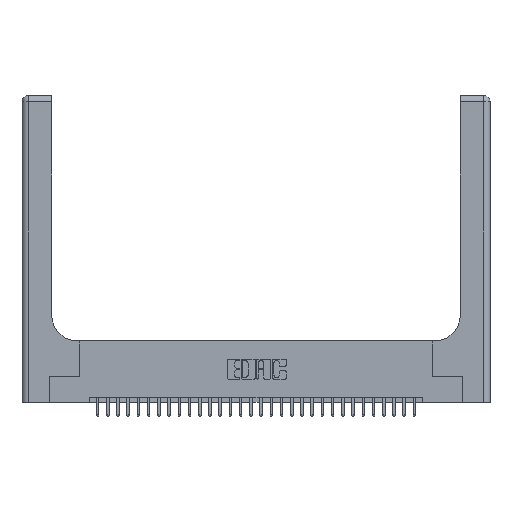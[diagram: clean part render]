
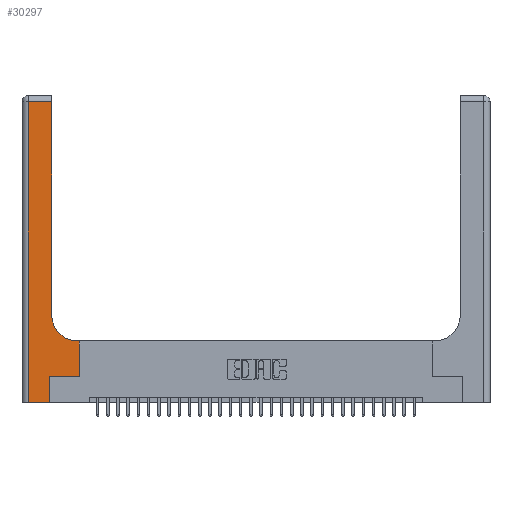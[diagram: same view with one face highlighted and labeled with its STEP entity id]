
A CAD part, top view. The second image highlights one B-rep face of the part: STEP entity #30297.
In plain terms, the highlighted planar face has unit normal (0, 0, 1).
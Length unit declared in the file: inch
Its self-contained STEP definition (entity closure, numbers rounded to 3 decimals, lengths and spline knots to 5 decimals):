
#451 = CARTESIAN_POINT ( 'NONE',  ( 0.06, 0., 0.37 ) ) ;
#680 = EDGE_CURVE ( 'NONE', #16066, #14403, #4061, .T. ) ;
#1610 = CARTESIAN_POINT ( 'NONE',  ( 0., 3., 0.37 ) ) ;
#1974 = ORIENTED_EDGE ( 'NONE', *, *, #22517, .T. ) ;
#2512 = CARTESIAN_POINT ( 'NONE',  ( 0.269, 0.25, 0.37 ) ) ;
#2565 = EDGE_CURVE ( 'NONE', #5691, #30309, #18176, .T. ) ;
#2757 = VERTEX_POINT ( 'NONE', #10152 ) ;
#2891 = EDGE_CURVE ( 'NONE', #23864, #22957, #27853, .T. ) ;
#3194 = VECTOR ( 'NONE', #7421, 39.37008 ) ;
#3577 = EDGE_CURVE ( 'NONE', #22957, #16066, #4499, .T. ) ;
#3822 = FACE_OUTER_BOUND ( 'NONE', #22578, .T. ) ;
#4061 = LINE ( 'NONE', #12243, #22825 ) ;
#4499 = CIRCLE ( 'NONE', #15619, 0.25 ) ;
#4752 = LINE ( 'NONE', #30649, #11666 ) ;
#5093 = DIRECTION ( 'NONE',  ( 0., 1., 0. ) ) ;
#5436 = ORIENTED_EDGE ( 'NONE', *, *, #22120, .T. ) ;
#5691 = VERTEX_POINT ( 'NONE', #451 ) ;
#6523 = EDGE_CURVE ( 'NONE', #2757, #23864, #14977, .T. ) ;
#6579 = DIRECTION ( 'NONE',  ( -1., 0., 0. ) ) ;
#7201 = DIRECTION ( 'NONE',  ( 1., 0., 0. ) ) ;
#7208 = CARTESIAN_POINT ( 'NONE',  ( 0.2915, 0.6, 0.37 ) ) ;
#7421 = DIRECTION ( 'NONE',  ( 1., 0., 0. ) ) ;
#7479 = ORIENTED_EDGE ( 'NONE', *, *, #6523, .T. ) ;
#7613 = VECTOR ( 'NONE', #19084, 39.37008 ) ;
#8499 = VECTOR ( 'NONE', #5093, 39.37008 ) ;
#9966 = DIRECTION ( 'NONE',  ( 0., 1., 0. ) ) ;
#10152 = CARTESIAN_POINT ( 'NONE',  ( 0.5585, 0.25, 0.37 ) ) ;
#11666 = VECTOR ( 'NONE', #6579, 39.37008 ) ;
#11760 = VERTEX_POINT ( 'NONE', #12774 ) ;
#12076 = ORIENTED_EDGE ( 'NONE', *, *, #16499, .T. ) ;
#12243 = CARTESIAN_POINT ( 'NONE',  ( 0.2915, 3., 0.37 ) ) ;
#12272 = ORIENTED_EDGE ( 'NONE', *, *, #3577, .T. ) ;
#12570 = DIRECTION ( 'NONE',  ( 0., 1., 0. ) ) ;
#12655 = CARTESIAN_POINT ( 'NONE',  ( 0.5415, 0.6, 0.37 ) ) ;
#12774 = CARTESIAN_POINT ( 'NONE',  ( 0.269, 0.25, 0.37 ) ) ;
#13090 = CARTESIAN_POINT ( 'NONE',  ( 0.2915, 0.85, 0.37 ) ) ;
#14183 = AXIS2_PLACEMENT_3D ( 'NONE', #1610, #25651, #28097 ) ;
#14403 = VERTEX_POINT ( 'NONE', #26130 ) ;
#14474 = CARTESIAN_POINT ( 'NONE',  ( 0., 0., 0.37 ) ) ;
#14977 = LINE ( 'NONE', #29488, #8499 ) ;
#15619 = AXIS2_PLACEMENT_3D ( 'NONE', #19596, #26948, #7201 ) ;
#16066 = VERTEX_POINT ( 'NONE', #13090 ) ;
#16219 = PLANE ( 'NONE',  #14183 ) ;
#16499 = EDGE_CURVE ( 'NONE', #11760, #2757, #31305, .T. ) ;
#17155 = CARTESIAN_POINT ( 'NONE',  ( 0.06, 2.94, 0.37 ) ) ;
#17859 = CARTESIAN_POINT ( 'NONE',  ( 0.5585, 0.6, 0.37 ) ) ;
#18176 = LINE ( 'NONE', #14474, #3194 ) ;
#19084 = DIRECTION ( 'NONE',  ( 0., -1., 0. ) ) ;
#19596 = CARTESIAN_POINT ( 'NONE',  ( 0.5415, 0.85, 0.37 ) ) ;
#19613 = DIRECTION ( 'NONE',  ( 1., 0., 0. ) ) ;
#20086 = ORIENTED_EDGE ( 'NONE', *, *, #2891, .T. ) ;
#21395 = VECTOR ( 'NONE', #29879, 39.37008 ) ;
#21410 = LINE ( 'NONE', #23253, #7613 ) ;
#21861 = ORIENTED_EDGE ( 'NONE', *, *, #680, .T. ) ;
#22120 = EDGE_CURVE ( 'NONE', #27079, #5691, #21410, .T. ) ;
#22517 = EDGE_CURVE ( 'NONE', #14403, #27079, #4752, .T. ) ;
#22578 = EDGE_LOOP ( 'NONE', ( #21861, #1974, #5436, #27131, #25622, #12076, #7479, #20086, #12272 ) ) ;
#22825 = VECTOR ( 'NONE', #12570, 39.37008 ) ;
#22957 = VERTEX_POINT ( 'NONE', #12655 ) ;
#23253 = CARTESIAN_POINT ( 'NONE',  ( 0.06, 3., 0.37 ) ) ;
#23864 = VERTEX_POINT ( 'NONE', #17859 ) ;
#24306 = LINE ( 'NONE', #26800, #29297 ) ;
#24810 = VECTOR ( 'NONE', #19613, 39.37008 ) ;
#25622 = ORIENTED_EDGE ( 'NONE', *, *, #28716, .T. ) ;
#25651 = DIRECTION ( 'NONE',  ( 0., 0., -1. ) ) ;
#26130 = CARTESIAN_POINT ( 'NONE',  ( 0.2915, 2.94, 0.37 ) ) ;
#26800 = CARTESIAN_POINT ( 'NONE',  ( 0.269, 0., 0.37 ) ) ;
#26948 = DIRECTION ( 'NONE',  ( 0., 0., -1. ) ) ;
#27079 = VERTEX_POINT ( 'NONE', #17155 ) ;
#27131 = ORIENTED_EDGE ( 'NONE', *, *, #2565, .T. ) ;
#27853 = LINE ( 'NONE', #7208, #21395 ) ;
#28097 = DIRECTION ( 'NONE',  ( -1., 0., 0. ) ) ;
#28549 = CARTESIAN_POINT ( 'NONE',  ( 0.269, 0., 0.37 ) ) ;
#28716 = EDGE_CURVE ( 'NONE', #30309, #11760, #24306, .T. ) ;
#29297 = VECTOR ( 'NONE', #9966, 39.37008 ) ;
#29488 = CARTESIAN_POINT ( 'NONE',  ( 0.5585, 0.25, 0.37 ) ) ;
#29879 = DIRECTION ( 'NONE',  ( -1., 0., 0. ) ) ;
#30297 = ADVANCED_FACE ( 'NONE', ( #3822 ), #16219, .F. ) ;
#30309 = VERTEX_POINT ( 'NONE', #28549 ) ;
#30649 = CARTESIAN_POINT ( 'NONE',  ( 0., 2.94, 0.37 ) ) ;
#31305 = LINE ( 'NONE', #2512, #24810 ) ;
